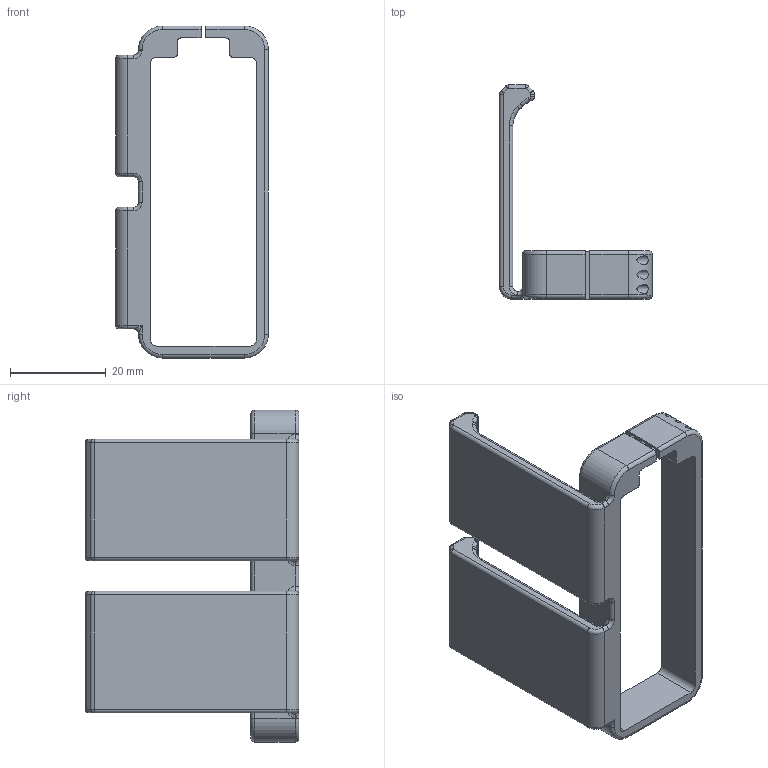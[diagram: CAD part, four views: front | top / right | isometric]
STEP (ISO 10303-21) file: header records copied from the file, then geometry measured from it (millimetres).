
FILE_DESCRIPTION (( 'STEP AP214' ), '1' );
FILE_NAME ('Filament_Clamp.STEP', '2013-12-11T18:01:57', ( 'elpi' ), ( '' ), 'SwSTEP 2.0', 'SolidWorks 2013', '' );
FILE_SCHEMA (( 'AUTOMOTIVE_DESIGN' ));
Length unit declared in the file: millimetre
Products named in the file (1): Filament_Clamp
Bounding box: 31.86 x 44.6 x 69.26 mm (x, y, z)
Volume: 11845.8 mm3; surface area: 10171 mm2
Topology: 1 solids, 1 shells, 183 faces, 438 edges, 259 vertices
Faces by surface type: cylinder 90, torus 51, plane 41, bspline 1
Entity records: 5476 total; most frequent: CARTESIAN_POINT 1044, DIRECTION 1029, ORIENTED_EDGE 874, EDGE_CURVE 437, AXIS2_PLACEMENT_3D 418, VERTEX_POINT 259, CIRCLE 235, VECTOR 193
